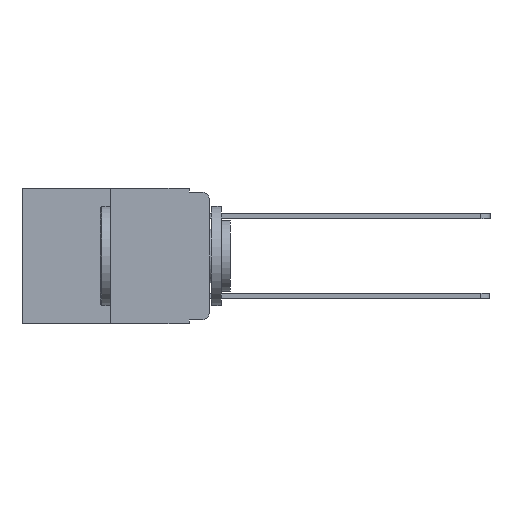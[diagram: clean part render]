
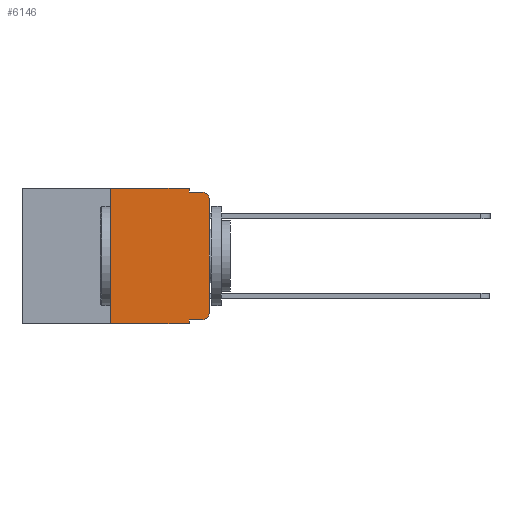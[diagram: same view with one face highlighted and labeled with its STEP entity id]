
A CAD part, left-side view. The second image highlights one B-rep face of the part: STEP entity #6146.
In plain terms, the highlighted planar face has unit normal (-1, 0, 0).
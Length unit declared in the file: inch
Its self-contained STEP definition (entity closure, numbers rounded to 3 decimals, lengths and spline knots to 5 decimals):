
#223 = CARTESIAN_POINT ( 'NONE',  ( 0., 0.051, -0.343 ) ) ;
#312 = CARTESIAN_POINT ( 'NONE',  ( 0., 0., -0.03 ) ) ;
#771 = DIRECTION ( 'NONE',  ( -1., 0., 0. ) ) ;
#923 = EDGE_CURVE ( 'NONE', #10335, #7524, #1738, .T. ) ;
#988 = VECTOR ( 'NONE', #8726, 39.37008 ) ;
#1135 = CARTESIAN_POINT ( 'NONE',  ( 0., 0.051, 0. ) ) ;
#1193 = VECTOR ( 'NONE', #11318, 39.37008 ) ;
#1217 = AXIS2_PLACEMENT_3D ( 'NONE', #8114, #11666, #6245 ) ;
#1271 = LINE ( 'NONE', #2580, #6082 ) ;
#1391 = DIRECTION ( 'NONE',  ( 0., -1., 0. ) ) ;
#1414 = LINE ( 'NONE', #7734, #3706 ) ;
#1674 = VECTOR ( 'NONE', #10018, 39.37008 ) ;
#1733 = CARTESIAN_POINT ( 'NONE',  ( 0., 0.25, -0.343 ) ) ;
#1738 = LINE ( 'NONE', #9369, #2338 ) ;
#1862 = ORIENTED_EDGE ( 'NONE', *, *, #2055, .T. ) ;
#1883 = EDGE_CURVE ( 'NONE', #4738, #8111, #1414, .T. ) ;
#2055 = EDGE_CURVE ( 'NONE', #5408, #7524, #2144, .T. ) ;
#2095 = DIRECTION ( 'NONE',  ( 0., 0., -1. ) ) ;
#2144 = CIRCLE ( 'NONE', #8590, 0.02 ) ;
#2338 = VECTOR ( 'NONE', #11613, 39.37008 ) ;
#2471 = ORIENTED_EDGE ( 'NONE', *, *, #1883, .T. ) ;
#2580 = CARTESIAN_POINT ( 'NONE',  ( 0., 0.25, 0. ) ) ;
#2675 = AXIS2_PLACEMENT_3D ( 'NONE', #6533, #771, #7494 ) ;
#3025 = VERTEX_POINT ( 'NONE', #223 ) ;
#3090 = ORIENTED_EDGE ( 'NONE', *, *, #923, .F. ) ;
#3706 = VECTOR ( 'NONE', #1391, 39.37008 ) ;
#3719 = ORIENTED_EDGE ( 'NONE', *, *, #4581, .T. ) ;
#3859 = ORIENTED_EDGE ( 'NONE', *, *, #9151, .T. ) ;
#4011 = CARTESIAN_POINT ( 'NONE',  ( 0., 0.473, 0. ) ) ;
#4183 = EDGE_CURVE ( 'NONE', #6331, #9665, #8880, .T. ) ;
#4555 = DIRECTION ( 'NONE',  ( 0., 0., 1. ) ) ;
#4581 = EDGE_CURVE ( 'NONE', #8111, #10163, #6987, .T. ) ;
#4691 = CARTESIAN_POINT ( 'NONE',  ( 0., 0.051, 0. ) ) ;
#4738 = VERTEX_POINT ( 'NONE', #11295 ) ;
#5088 = EDGE_CURVE ( 'NONE', #5176, #6331, #1271, .T. ) ;
#5176 = VERTEX_POINT ( 'NONE', #1733 ) ;
#5293 = EDGE_CURVE ( 'NONE', #9665, #10335, #9280, .T. ) ;
#5303 = PLANE ( 'NONE',  #1217 ) ;
#5408 = VERTEX_POINT ( 'NONE', #312 ) ;
#5627 = ORIENTED_EDGE ( 'NONE', *, *, #5293, .F. ) ;
#5872 = EDGE_LOOP ( 'NONE', ( #6068, #1862, #3090, #5627, #8693, #10909, #3859, #11471, #2471, #3719 ) ) ;
#6068 = ORIENTED_EDGE ( 'NONE', *, *, #6384, .T. ) ;
#6082 = VECTOR ( 'NONE', #4555, 39.37008 ) ;
#6146 = ADVANCED_FACE ( 'NONE', ( #9939 ), #5303, .F. ) ;
#6231 = VECTOR ( 'NONE', #2095, 39.37008 ) ;
#6245 = DIRECTION ( 'NONE',  ( 0., 0., -1. ) ) ;
#6303 = LINE ( 'NONE', #10441, #1193 ) ;
#6331 = VERTEX_POINT ( 'NONE', #6490 ) ;
#6384 = EDGE_CURVE ( 'NONE', #10163, #5408, #10612, .T. ) ;
#6490 = CARTESIAN_POINT ( 'NONE',  ( 0., 0.25, 0. ) ) ;
#6533 = CARTESIAN_POINT ( 'NONE',  ( 0., 0.02, -0.313 ) ) ;
#6987 = CIRCLE ( 'NONE', #2675, 0.02 ) ;
#7494 = DIRECTION ( 'NONE',  ( 0., 0., -1. ) ) ;
#7524 = VERTEX_POINT ( 'NONE', #10784 ) ;
#7594 = EDGE_CURVE ( 'NONE', #4738, #3025, #9238, .T. ) ;
#7734 = CARTESIAN_POINT ( 'NONE',  ( 0., 0.051, -0.333 ) ) ;
#8111 = VERTEX_POINT ( 'NONE', #11548 ) ;
#8114 = CARTESIAN_POINT ( 'NONE',  ( 0., 0.473, 0. ) ) ;
#8483 = CARTESIAN_POINT ( 'NONE',  ( 0., 0.051, -0.01 ) ) ;
#8590 = AXIS2_PLACEMENT_3D ( 'NONE', #8747, #11877, #10395 ) ;
#8693 = ORIENTED_EDGE ( 'NONE', *, *, #4183, .F. ) ;
#8726 = DIRECTION ( 'NONE',  ( 0., -1., 0. ) ) ;
#8747 = CARTESIAN_POINT ( 'NONE',  ( 0., 0.02, -0.03 ) ) ;
#8880 = LINE ( 'NONE', #4011, #988 ) ;
#9151 = EDGE_CURVE ( 'NONE', #5176, #3025, #6303, .T. ) ;
#9238 = LINE ( 'NONE', #10887, #1674 ) ;
#9280 = LINE ( 'NONE', #1135, #6231 ) ;
#9369 = CARTESIAN_POINT ( 'NONE',  ( 0., 0.051, -0.01 ) ) ;
#9665 = VERTEX_POINT ( 'NONE', #4691 ) ;
#9939 = FACE_OUTER_BOUND ( 'NONE', #5872, .T. ) ;
#10018 = DIRECTION ( 'NONE',  ( 0., 0., -1. ) ) ;
#10047 = CARTESIAN_POINT ( 'NONE',  ( 0., 0., -0.313 ) ) ;
#10062 = VECTOR ( 'NONE', #11067, 39.37008 ) ;
#10163 = VERTEX_POINT ( 'NONE', #10047 ) ;
#10206 = CARTESIAN_POINT ( 'NONE',  ( 0., 0., 0. ) ) ;
#10335 = VERTEX_POINT ( 'NONE', #8483 ) ;
#10395 = DIRECTION ( 'NONE',  ( 0., 0., -1. ) ) ;
#10441 = CARTESIAN_POINT ( 'NONE',  ( 0., 0.473, -0.343 ) ) ;
#10612 = LINE ( 'NONE', #10206, #10062 ) ;
#10784 = CARTESIAN_POINT ( 'NONE',  ( 0., 0.02, -0.01 ) ) ;
#10887 = CARTESIAN_POINT ( 'NONE',  ( 0., 0.051, 0. ) ) ;
#10909 = ORIENTED_EDGE ( 'NONE', *, *, #5088, .F. ) ;
#11067 = DIRECTION ( 'NONE',  ( 0., 0., 1. ) ) ;
#11295 = CARTESIAN_POINT ( 'NONE',  ( 0., 0.051, -0.333 ) ) ;
#11318 = DIRECTION ( 'NONE',  ( 0., -1., 0. ) ) ;
#11471 = ORIENTED_EDGE ( 'NONE', *, *, #7594, .F. ) ;
#11548 = CARTESIAN_POINT ( 'NONE',  ( 0., 0.02, -0.333 ) ) ;
#11613 = DIRECTION ( 'NONE',  ( 0., -1., 0. ) ) ;
#11666 = DIRECTION ( 'NONE',  ( 1., 0., 0. ) ) ;
#11877 = DIRECTION ( 'NONE',  ( -1., 0., 0. ) ) ;
